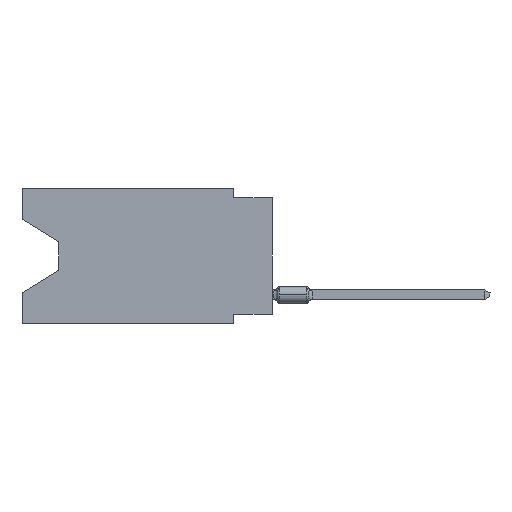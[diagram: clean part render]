
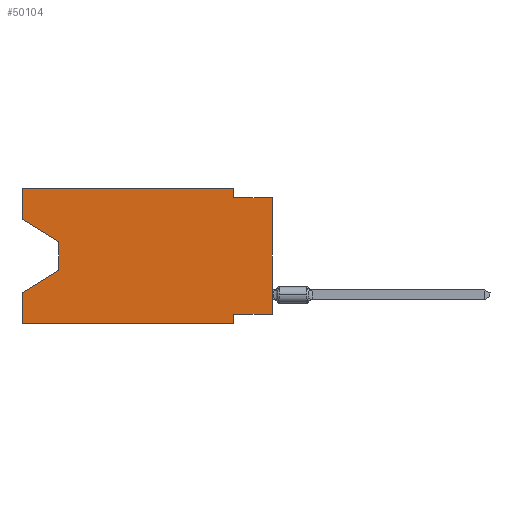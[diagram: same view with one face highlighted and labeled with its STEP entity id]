
A CAD part, left-side view. The second image highlights one B-rep face of the part: STEP entity #50104.
In plain terms, the highlighted planar face has unit normal (-1, 0, 0).
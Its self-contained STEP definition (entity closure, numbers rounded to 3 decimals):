
#1563 = LINE ( 'NONE', #40813, #30562 ) ;
#2104 = LINE ( 'NONE', #47327, #20988 ) ;
#3917 = ORIENTED_EDGE ( 'NONE', *, *, #72258, .T. ) ;
#3967 = VECTOR ( 'NONE', #50038, 1000. ) ;
#3992 = ORIENTED_EDGE ( 'NONE', *, *, #24660, .F. ) ;
#4075 = VECTOR ( 'NONE', #4496, 1000. ) ;
#4097 = ORIENTED_EDGE ( 'NONE', *, *, #64652, .T. ) ;
#4369 = LINE ( 'NONE', #72772, #58732 ) ;
#4496 = DIRECTION ( 'NONE',  ( 0., 0., 1. ) ) ;
#4848 = DIRECTION ( 'NONE',  ( 0., 0.855, -0.519 ) ) ;
#4860 = LINE ( 'NONE', #8999, #4075 ) ;
#7911 = DIRECTION ( 'NONE',  ( 0., 1., 0. ) ) ;
#8999 = CARTESIAN_POINT ( 'NONE',  ( 0., 16.383, 0. ) ) ;
#9108 = CARTESIAN_POINT ( 'NONE',  ( 0., 0., -8.255 ) ) ;
#9731 = CARTESIAN_POINT ( 'NONE',  ( 0., 0., -0.635 ) ) ;
#12696 = VECTOR ( 'NONE', #15953, 1000. ) ;
#14021 = VERTEX_POINT ( 'NONE', #38937 ) ;
#14280 = CARTESIAN_POINT ( 'NONE',  ( 0., 0., 0. ) ) ;
#15953 = DIRECTION ( 'NONE',  ( 0., 0., -1. ) ) ;
#16383 = CARTESIAN_POINT ( 'NONE',  ( 0., 2.54, -8.89 ) ) ;
#18481 = EDGE_CURVE ( 'NONE', #14021, #37632, #4369, .T. ) ;
#18761 = VERTEX_POINT ( 'NONE', #64876 ) ;
#19356 = CARTESIAN_POINT ( 'NONE',  ( 0., 16.383, 0. ) ) ;
#20067 = VECTOR ( 'NONE', #33562, 1000. ) ;
#20851 = EDGE_CURVE ( 'NONE', #38698, #71877, #4860, .T. ) ;
#20988 = VECTOR ( 'NONE', #46962, 1000. ) ;
#22074 = CARTESIAN_POINT ( 'NONE',  ( 0., 16.383, -6.852 ) ) ;
#22958 = EDGE_CURVE ( 'NONE', #18761, #55893, #73596, .T. ) ;
#23911 = VECTOR ( 'NONE', #72940, 1000. ) ;
#24660 = EDGE_CURVE ( 'NONE', #68305, #71560, #67911, .T. ) ;
#29072 = ORIENTED_EDGE ( 'NONE', *, *, #20851, .F. ) ;
#30562 = VECTOR ( 'NONE', #7911, 1000. ) ;
#31102 = EDGE_CURVE ( 'NONE', #71877, #68305, #70577, .T. ) ;
#32324 = EDGE_CURVE ( 'NONE', #71560, #72838, #38495, .T. ) ;
#32491 = VECTOR ( 'NONE', #4848, 1000. ) ;
#32607 = EDGE_CURVE ( 'NONE', #55893, #37840, #35086, .T. ) ;
#33562 = DIRECTION ( 'NONE',  ( 0., 0., -1. ) ) ;
#33834 = CARTESIAN_POINT ( 'NONE',  ( 0., 16.383, -2.038 ) ) ;
#35086 = LINE ( 'NONE', #45209, #32491 ) ;
#35153 = VECTOR ( 'NONE', #72841, 1000. ) ;
#37632 = VERTEX_POINT ( 'NONE', #70357 ) ;
#37763 = EDGE_LOOP ( 'NONE', ( #3917, #48274, #64785, #39125, #61249, #72657, #58348, #4097, #50258, #3992, #54447, #29072 ) ) ;
#37840 = VERTEX_POINT ( 'NONE', #22074 ) ;
#38227 = EDGE_CURVE ( 'NONE', #47023, #37632, #49296, .T. ) ;
#38495 = LINE ( 'NONE', #9731, #59884 ) ;
#38698 = VERTEX_POINT ( 'NONE', #33834 ) ;
#38824 = CARTESIAN_POINT ( 'NONE',  ( 0., 16.383, 0. ) ) ;
#38937 = CARTESIAN_POINT ( 'NONE',  ( 0., 16.383, -8.89 ) ) ;
#39125 = ORIENTED_EDGE ( 'NONE', *, *, #42933, .F. ) ;
#39477 = DIRECTION ( 'NONE',  ( 0., -1., 0. ) ) ;
#39545 = LINE ( 'NONE', #38824, #3967 ) ;
#40813 = CARTESIAN_POINT ( 'NONE',  ( 0., 0., -8.255 ) ) ;
#41101 = FACE_OUTER_BOUND ( 'NONE', #37763, .T. ) ;
#42933 = EDGE_CURVE ( 'NONE', #14021, #37840, #39545, .T. ) ;
#42983 = AXIS2_PLACEMENT_3D ( 'NONE', #58671, #53049, #63900 ) ;
#45050 = EDGE_CURVE ( 'NONE', #46478, #47023, #1563, .T. ) ;
#45209 = CARTESIAN_POINT ( 'NONE',  ( 0., 13.97, -5.385 ) ) ;
#46478 = VERTEX_POINT ( 'NONE', #9108 ) ;
#46556 = CARTESIAN_POINT ( 'NONE',  ( 0., 13.97, -5.385 ) ) ;
#46962 = DIRECTION ( 'NONE',  ( 0., -0.855, -0.519 ) ) ;
#47023 = VERTEX_POINT ( 'NONE', #56368 ) ;
#47327 = CARTESIAN_POINT ( 'NONE',  ( 0., 16.383, -2.038 ) ) ;
#48274 = ORIENTED_EDGE ( 'NONE', *, *, #22958, .T. ) ;
#49036 = LINE ( 'NONE', #14280, #23911 ) ;
#49296 = LINE ( 'NONE', #16383, #20067 ) ;
#49349 = CARTESIAN_POINT ( 'NONE',  ( 0., 0., -0.635 ) ) ;
#50038 = DIRECTION ( 'NONE',  ( 0., 0., 1. ) ) ;
#50040 = CARTESIAN_POINT ( 'NONE',  ( 0., 13.97, -3.505 ) ) ;
#50104 = ADVANCED_FACE ( 'NONE', ( #41101 ), #58299, .F. ) ;
#50258 = ORIENTED_EDGE ( 'NONE', *, *, #32324, .F. ) ;
#50438 = VECTOR ( 'NONE', #65704, 1000. ) ;
#53049 = DIRECTION ( 'NONE',  ( 1., 0., 0. ) ) ;
#54447 = ORIENTED_EDGE ( 'NONE', *, *, #31102, .F. ) ;
#54860 = CARTESIAN_POINT ( 'NONE',  ( 0., 2.54, -0.635 ) ) ;
#55893 = VERTEX_POINT ( 'NONE', #46556 ) ;
#56368 = CARTESIAN_POINT ( 'NONE',  ( 0., 2.54, -8.255 ) ) ;
#58299 = PLANE ( 'NONE',  #42983 ) ;
#58348 = ORIENTED_EDGE ( 'NONE', *, *, #45050, .F. ) ;
#58671 = CARTESIAN_POINT ( 'NONE',  ( 0., 16.383, 0. ) ) ;
#58732 = VECTOR ( 'NONE', #39477, 1000. ) ;
#59884 = VECTOR ( 'NONE', #60206, 1000. ) ;
#60161 = CARTESIAN_POINT ( 'NONE',  ( 0., 2.54, 0. ) ) ;
#60206 = DIRECTION ( 'NONE',  ( 0., -1., 0. ) ) ;
#61249 = ORIENTED_EDGE ( 'NONE', *, *, #18481, .T. ) ;
#63900 = DIRECTION ( 'NONE',  ( 0., 0., -1. ) ) ;
#64652 = EDGE_CURVE ( 'NONE', #46478, #72838, #49036, .T. ) ;
#64785 = ORIENTED_EDGE ( 'NONE', *, *, #32607, .T. ) ;
#64876 = CARTESIAN_POINT ( 'NONE',  ( 0., 13.97, -3.505 ) ) ;
#65704 = DIRECTION ( 'NONE',  ( 0., -1., 0. ) ) ;
#67911 = LINE ( 'NONE', #72028, #12696 ) ;
#68305 = VERTEX_POINT ( 'NONE', #60161 ) ;
#69034 = CARTESIAN_POINT ( 'NONE',  ( 0., 16.383, 0. ) ) ;
#70357 = CARTESIAN_POINT ( 'NONE',  ( 0., 2.54, -8.89 ) ) ;
#70577 = LINE ( 'NONE', #19356, #50438 ) ;
#71560 = VERTEX_POINT ( 'NONE', #54860 ) ;
#71877 = VERTEX_POINT ( 'NONE', #69034 ) ;
#72028 = CARTESIAN_POINT ( 'NONE',  ( 0., 2.54, 0. ) ) ;
#72258 = EDGE_CURVE ( 'NONE', #38698, #18761, #2104, .T. ) ;
#72657 = ORIENTED_EDGE ( 'NONE', *, *, #38227, .F. ) ;
#72772 = CARTESIAN_POINT ( 'NONE',  ( 0., 16.383, -8.89 ) ) ;
#72838 = VERTEX_POINT ( 'NONE', #49349 ) ;
#72841 = DIRECTION ( 'NONE',  ( 0., 0., -1. ) ) ;
#72940 = DIRECTION ( 'NONE',  ( 0., 0., 1. ) ) ;
#73596 = LINE ( 'NONE', #50040, #35153 ) ;
